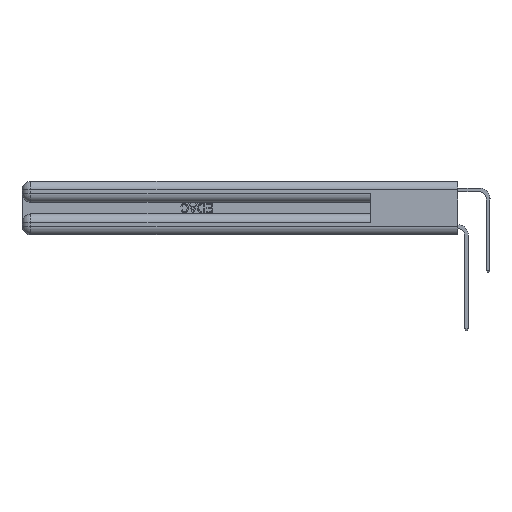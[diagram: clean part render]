
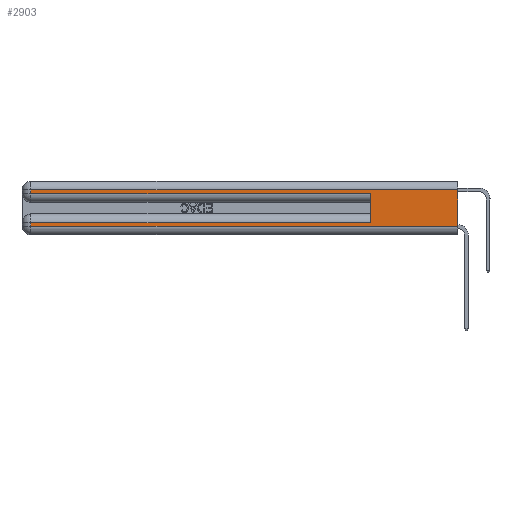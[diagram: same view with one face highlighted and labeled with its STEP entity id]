
A CAD part, left-side view. The second image highlights one B-rep face of the part: STEP entity #2903.
In plain terms, the highlighted planar face has unit normal (-1, 0, 0).
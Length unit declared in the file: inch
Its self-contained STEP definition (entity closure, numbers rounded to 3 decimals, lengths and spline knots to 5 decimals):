
#2 = CARTESIAN_POINT ( 'NONE',  ( 0., 0., 0.31 ) ) ;
#238 = ORIENTED_EDGE ( 'NONE', *, *, #13615, .T. ) ;
#1335 = FACE_OUTER_BOUND ( 'NONE', #26102, .T. ) ;
#1580 = CARTESIAN_POINT ( 'NONE',  ( 0., 0., 0.06 ) ) ;
#2521 = ORIENTED_EDGE ( 'NONE', *, *, #28003, .T. ) ;
#2903 = ADVANCED_FACE ( 'NONE', ( #1335 ), #21897, .F. ) ;
#3097 = VERTEX_POINT ( 'NONE', #3613 ) ;
#3613 = CARTESIAN_POINT ( 'NONE',  ( 0., 0.6, 0.285 ) ) ;
#3959 = DIRECTION ( 'NONE',  ( 0., 1., 0. ) ) ;
#5290 = VECTOR ( 'NONE', #22914, 39.37008 ) ;
#5416 = CARTESIAN_POINT ( 'NONE',  ( 0., 0., 0.085 ) ) ;
#5789 = VERTEX_POINT ( 'NONE', #18549 ) ;
#5953 = LINE ( 'NONE', #10290, #15706 ) ;
#6167 = CARTESIAN_POINT ( 'NONE',  ( 0., 0., 0.31 ) ) ;
#6738 = VECTOR ( 'NONE', #3959, 39.37008 ) ;
#6748 = EDGE_CURVE ( 'NONE', #5789, #17268, #18426, .T. ) ;
#8348 = CARTESIAN_POINT ( 'NONE',  ( 0., 0., 0.37 ) ) ;
#10135 = CARTESIAN_POINT ( 'NONE',  ( 0., 2.94, 0.37 ) ) ;
#10290 = CARTESIAN_POINT ( 'NONE',  ( 0., 0., 0.285 ) ) ;
#10588 = EDGE_CURVE ( 'NONE', #17268, #25922, #27916, .T. ) ;
#11120 = VECTOR ( 'NONE', #26090, 39.37008 ) ;
#13615 = EDGE_CURVE ( 'NONE', #24091, #3097, #5953, .T. ) ;
#13648 = LINE ( 'NONE', #16855, #11120 ) ;
#13782 = ORIENTED_EDGE ( 'NONE', *, *, #21063, .F. ) ;
#14835 = VECTOR ( 'NONE', #26225, 39.37008 ) ;
#14977 = VERTEX_POINT ( 'NONE', #1580 ) ;
#15706 = VECTOR ( 'NONE', #21430, 39.37008 ) ;
#16259 = VERTEX_POINT ( 'NONE', #2 ) ;
#16294 = CARTESIAN_POINT ( 'NONE',  ( 0., 2.94, 0.37 ) ) ;
#16331 = ORIENTED_EDGE ( 'NONE', *, *, #27819, .T. ) ;
#16855 = CARTESIAN_POINT ( 'NONE',  ( 0., 0., 0.37 ) ) ;
#17202 = DIRECTION ( 'NONE',  ( 0., 0., -1. ) ) ;
#17215 = EDGE_CURVE ( 'NONE', #25922, #14977, #25526, .T. ) ;
#17268 = VERTEX_POINT ( 'NONE', #28655 ) ;
#18131 = ORIENTED_EDGE ( 'NONE', *, *, #24734, .F. ) ;
#18426 = LINE ( 'NONE', #5416, #14835 ) ;
#18549 = CARTESIAN_POINT ( 'NONE',  ( 0., 0.6, 0.085 ) ) ;
#19589 = ORIENTED_EDGE ( 'NONE', *, *, #6748, .T. ) ;
#19593 = CARTESIAN_POINT ( 'NONE',  ( 0., 2.94, 0.06 ) ) ;
#20014 = AXIS2_PLACEMENT_3D ( 'NONE', #8348, #24441, #26623 ) ;
#21009 = VERTEX_POINT ( 'NONE', #21449 ) ;
#21063 = EDGE_CURVE ( 'NONE', #16259, #14977, #13648, .T. ) ;
#21430 = DIRECTION ( 'NONE',  ( 0., -1., 0. ) ) ;
#21449 = CARTESIAN_POINT ( 'NONE',  ( 0., 2.94, 0.31 ) ) ;
#21646 = CARTESIAN_POINT ( 'NONE',  ( 0., 0., 0.06 ) ) ;
#21825 = VECTOR ( 'NONE', #17202, 39.37008 ) ;
#21897 = PLANE ( 'NONE',  #20014 ) ;
#22914 = DIRECTION ( 'NONE',  ( 0., 0., -1. ) ) ;
#23799 = CARTESIAN_POINT ( 'NONE',  ( 0., 0.6, 0.145 ) ) ;
#24091 = VERTEX_POINT ( 'NONE', #28434 ) ;
#24441 = DIRECTION ( 'NONE',  ( 1., 0., 0. ) ) ;
#24497 = DIRECTION ( 'NONE',  ( 0., 0., 1. ) ) ;
#24734 = EDGE_CURVE ( 'NONE', #5789, #3097, #25244, .T. ) ;
#25060 = LINE ( 'NONE', #6167, #6738 ) ;
#25244 = LINE ( 'NONE', #23799, #27729 ) ;
#25394 = LINE ( 'NONE', #16294, #5290 ) ;
#25526 = LINE ( 'NONE', #21646, #26252 ) ;
#25922 = VERTEX_POINT ( 'NONE', #19593 ) ;
#26090 = DIRECTION ( 'NONE',  ( 0., 0., -1. ) ) ;
#26102 = EDGE_LOOP ( 'NONE', ( #13782, #16331, #2521, #238, #18131, #19589, #28084, #26617 ) ) ;
#26225 = DIRECTION ( 'NONE',  ( 0., 1., 0. ) ) ;
#26252 = VECTOR ( 'NONE', #28852, 39.37008 ) ;
#26617 = ORIENTED_EDGE ( 'NONE', *, *, #17215, .T. ) ;
#26623 = DIRECTION ( 'NONE',  ( 0., 0., -1. ) ) ;
#27729 = VECTOR ( 'NONE', #24497, 39.37008 ) ;
#27819 = EDGE_CURVE ( 'NONE', #16259, #21009, #25060, .T. ) ;
#27916 = LINE ( 'NONE', #10135, #21825 ) ;
#28003 = EDGE_CURVE ( 'NONE', #21009, #24091, #25394, .T. ) ;
#28084 = ORIENTED_EDGE ( 'NONE', *, *, #10588, .T. ) ;
#28434 = CARTESIAN_POINT ( 'NONE',  ( 0., 2.94, 0.285 ) ) ;
#28655 = CARTESIAN_POINT ( 'NONE',  ( 0., 2.94, 0.085 ) ) ;
#28852 = DIRECTION ( 'NONE',  ( 0., -1., 0. ) ) ;
